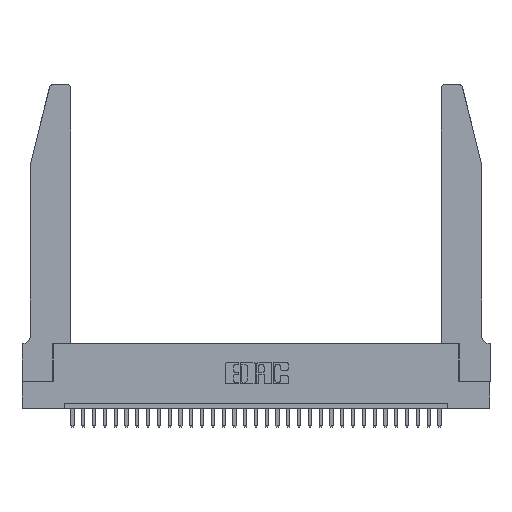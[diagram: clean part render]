
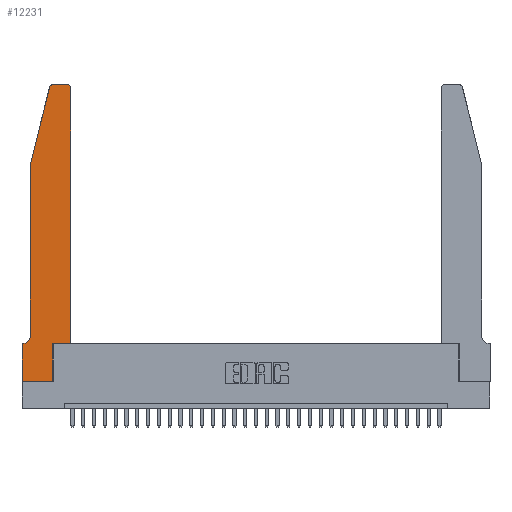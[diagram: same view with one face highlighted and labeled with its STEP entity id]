
A CAD part, top view. The second image highlights one B-rep face of the part: STEP entity #12231.
In plain terms, the highlighted planar face has unit normal (0, 0, 1).
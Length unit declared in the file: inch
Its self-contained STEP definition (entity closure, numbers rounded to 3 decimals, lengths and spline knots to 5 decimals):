
#140 = VECTOR ( 'NONE', #22412, 39.37008 ) ;
#575 = LINE ( 'NONE', #23973, #6387 ) ;
#655 = CARTESIAN_POINT ( 'NONE',  ( 0.4205, 2.75, 0.37 ) ) ;
#659 = CARTESIAN_POINT ( 'NONE',  ( 0.0055, 0.42, 0.37 ) ) ;
#684 = VECTOR ( 'NONE', #31678, 39.37008 ) ;
#818 = LINE ( 'NONE', #3285, #11668 ) ;
#1248 = CARTESIAN_POINT ( 'NONE',  ( 0.2865, 0.35, 0.37 ) ) ;
#1856 = VERTEX_POINT ( 'NONE', #18717 ) ;
#2295 = EDGE_CURVE ( 'NONE', #7633, #24481, #22176, .T. ) ;
#2523 = LINE ( 'NONE', #13661, #2561 ) ;
#2561 = VECTOR ( 'NONE', #13866, 39.37008 ) ;
#2888 = CIRCLE ( 'NONE', #21943, 0.07 ) ;
#3281 = CARTESIAN_POINT ( 'NONE',  ( 0.2865, 0., 0.37 ) ) ;
#3285 = CARTESIAN_POINT ( 'NONE',  ( 0.0755, 2., 0.37 ) ) ;
#3962 = EDGE_CURVE ( 'NONE', #17298, #18271, #8950, .T. ) ;
#4444 = ORIENTED_EDGE ( 'NONE', *, *, #22932, .T. ) ;
#4519 = LINE ( 'NONE', #27623, #4920 ) ;
#4920 = VECTOR ( 'NONE', #30325, 39.37008 ) ;
#5194 = CARTESIAN_POINT ( 'NONE',  ( 0., 0.35, 0.37 ) ) ;
#5792 = EDGE_CURVE ( 'NONE', #1856, #11286, #4519, .T. ) ;
#5992 = DIRECTION ( 'NONE',  ( 0., 0., 1. ) ) ;
#6104 = CARTESIAN_POINT ( 'NONE',  ( 0.4205, 2.72, 0.37 ) ) ;
#6119 = VERTEX_POINT ( 'NONE', #16282 ) ;
#6188 = ORIENTED_EDGE ( 'NONE', *, *, #28148, .T. ) ;
#6219 = DIRECTION ( 'NONE',  ( 0., 1., 0. ) ) ;
#6387 = VECTOR ( 'NONE', #31271, 39.37008 ) ;
#7410 = CARTESIAN_POINT ( 'NONE',  ( 0.4505, 0.35, 0.37 ) ) ;
#7633 = VERTEX_POINT ( 'NONE', #20053 ) ;
#7680 = DIRECTION ( 'NONE',  ( 1., 0., 0. ) ) ;
#7900 = EDGE_CURVE ( 'NONE', #6119, #28101, #28480, .T. ) ;
#7930 = DIRECTION ( 'NONE',  ( 0., 0., -1. ) ) ;
#8287 = CARTESIAN_POINT ( 'NONE',  ( 0.0755, 0.42, 0.37 ) ) ;
#8299 = LINE ( 'NONE', #19812, #140 ) ;
#8394 = DIRECTION ( 'NONE',  ( 0., -1., 0. ) ) ;
#8950 = CIRCLE ( 'NONE', #8965, 0.03 ) ;
#8965 = AXIS2_PLACEMENT_3D ( 'NONE', #6104, #5992, #18238 ) ;
#9447 = CARTESIAN_POINT ( 'NONE',  ( 0., 0., 0.37 ) ) ;
#9452 = DIRECTION ( 'NONE',  ( 0., 0., 1. ) ) ;
#9970 = EDGE_CURVE ( 'NONE', #24481, #22059, #575, .T. ) ;
#10209 = EDGE_CURVE ( 'NONE', #29496, #22192, #2888, .T. ) ;
#10324 = DIRECTION ( 'NONE',  ( -1., 0., 0. ) ) ;
#10568 = CARTESIAN_POINT ( 'NONE',  ( 0.0755, 2., 0.37 ) ) ;
#10598 = VECTOR ( 'NONE', #6219, 39.37008 ) ;
#11286 = VERTEX_POINT ( 'NONE', #7410 ) ;
#11668 = VECTOR ( 'NONE', #8394, 39.37008 ) ;
#12159 = CARTESIAN_POINT ( 'NONE',  ( 0.284, 2.72, 0.37 ) ) ;
#12231 = ADVANCED_FACE ( 'NONE', ( #23317 ), #27348, .T. ) ;
#12337 = ORIENTED_EDGE ( 'NONE', *, *, #10209, .T. ) ;
#13661 = CARTESIAN_POINT ( 'NONE',  ( 0.2605, 2.75, 0.37 ) ) ;
#13866 = DIRECTION ( 'NONE',  ( -1., 0., 0. ) ) ;
#14292 = CARTESIAN_POINT ( 'NONE',  ( 0.0755, 0.35, 0.37 ) ) ;
#14327 = CARTESIAN_POINT ( 'NONE',  ( 0., 0., 0.37 ) ) ;
#14905 = CARTESIAN_POINT ( 'NONE',  ( 0.4505, 2.72, 0.37 ) ) ;
#15167 = DIRECTION ( 'NONE',  ( 1., 0., 0. ) ) ;
#16282 = CARTESIAN_POINT ( 'NONE',  ( 0., 0.35, 0.37 ) ) ;
#17042 = DIRECTION ( 'NONE',  ( 1., 0., 0. ) ) ;
#17093 = ORIENTED_EDGE ( 'NONE', *, *, #2295, .T. ) ;
#17298 = VERTEX_POINT ( 'NONE', #14905 ) ;
#17684 = ORIENTED_EDGE ( 'NONE', *, *, #28236, .T. ) ;
#17707 = EDGE_CURVE ( 'NONE', #22192, #6119, #23957, .T. ) ;
#18225 = CARTESIAN_POINT ( 'NONE',  ( 0.0055, 0.35, 0.37 ) ) ;
#18238 = DIRECTION ( 'NONE',  ( 1., 0., 0. ) ) ;
#18271 = VERTEX_POINT ( 'NONE', #655 ) ;
#18717 = CARTESIAN_POINT ( 'NONE',  ( 0.2865, 0.35, 0.37 ) ) ;
#19330 = VERTEX_POINT ( 'NONE', #3281 ) ;
#19440 = ORIENTED_EDGE ( 'NONE', *, *, #5792, .T. ) ;
#19812 = CARTESIAN_POINT ( 'NONE',  ( 0.4505, 0.35, 0.37 ) ) ;
#20053 = CARTESIAN_POINT ( 'NONE',  ( 0.284, 2.75, 0.37 ) ) ;
#20315 = EDGE_CURVE ( 'NONE', #11286, #17298, #8299, .T. ) ;
#21018 = ORIENTED_EDGE ( 'NONE', *, *, #3962, .T. ) ;
#21431 = LINE ( 'NONE', #14327, #28851 ) ;
#21943 = AXIS2_PLACEMENT_3D ( 'NONE', #659, #7930, #10324 ) ;
#22059 = VERTEX_POINT ( 'NONE', #10568 ) ;
#22176 = CIRCLE ( 'NONE', #23056, 0.03 ) ;
#22182 = CARTESIAN_POINT ( 'NONE',  ( 0.25487, 2.72718, 0.37 ) ) ;
#22192 = VERTEX_POINT ( 'NONE', #18225 ) ;
#22412 = DIRECTION ( 'NONE',  ( 0., 1., 0. ) ) ;
#22541 = DIRECTION ( 'NONE',  ( 0., 0., 1. ) ) ;
#22850 = ORIENTED_EDGE ( 'NONE', *, *, #9970, .T. ) ;
#22932 = EDGE_CURVE ( 'NONE', #18271, #7633, #2523, .T. ) ;
#23056 = AXIS2_PLACEMENT_3D ( 'NONE', #12159, #9452, #15167 ) ;
#23238 = AXIS2_PLACEMENT_3D ( 'NONE', #5194, #22541, #7680 ) ;
#23317 = FACE_OUTER_BOUND ( 'NONE', #23523, .T. ) ;
#23523 = EDGE_LOOP ( 'NONE', ( #4444, #17093, #22850, #28086, #12337, #24195, #26564, #17684, #6188, #19440, #27963, #21018 ) ) ;
#23957 = LINE ( 'NONE', #14292, #684 ) ;
#23973 = CARTESIAN_POINT ( 'NONE',  ( 0.0755, 2., 0.37 ) ) ;
#24195 = ORIENTED_EDGE ( 'NONE', *, *, #17707, .T. ) ;
#24481 = VERTEX_POINT ( 'NONE', #22182 ) ;
#26564 = ORIENTED_EDGE ( 'NONE', *, *, #7900, .T. ) ;
#27348 = PLANE ( 'NONE',  #23238 ) ;
#27623 = CARTESIAN_POINT ( 'NONE',  ( 0.4505, 0.35, 0.37 ) ) ;
#27963 = ORIENTED_EDGE ( 'NONE', *, *, #20315, .T. ) ;
#28086 = ORIENTED_EDGE ( 'NONE', *, *, #29443, .T. ) ;
#28101 = VERTEX_POINT ( 'NONE', #30964 ) ;
#28148 = EDGE_CURVE ( 'NONE', #19330, #1856, #31964, .T. ) ;
#28236 = EDGE_CURVE ( 'NONE', #28101, #19330, #21431, .T. ) ;
#28480 = LINE ( 'NONE', #9447, #29615 ) ;
#28851 = VECTOR ( 'NONE', #17042, 39.37008 ) ;
#29443 = EDGE_CURVE ( 'NONE', #22059, #29496, #818, .T. ) ;
#29496 = VERTEX_POINT ( 'NONE', #8287 ) ;
#29615 = VECTOR ( 'NONE', #31591, 39.37008 ) ;
#30325 = DIRECTION ( 'NONE',  ( 1., 0., 0. ) ) ;
#30964 = CARTESIAN_POINT ( 'NONE',  ( 0., 0., 0.37 ) ) ;
#31271 = DIRECTION ( 'NONE',  ( -0.239, -0.971, 0. ) ) ;
#31591 = DIRECTION ( 'NONE',  ( 0., -1., 0. ) ) ;
#31678 = DIRECTION ( 'NONE',  ( -1., 0., 0. ) ) ;
#31964 = LINE ( 'NONE', #1248, #10598 ) ;
